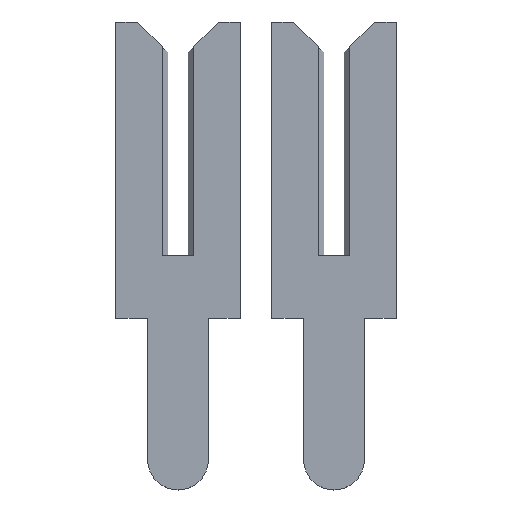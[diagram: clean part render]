
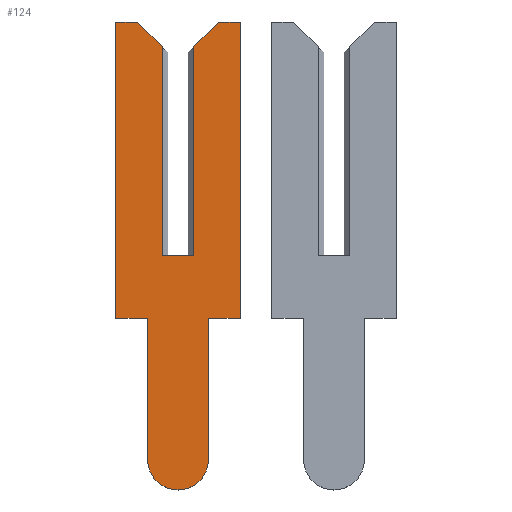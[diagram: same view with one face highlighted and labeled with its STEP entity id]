
A CAD part, top view. The second image highlights one B-rep face of the part: STEP entity #124.
In plain terms, the highlighted face is planar.
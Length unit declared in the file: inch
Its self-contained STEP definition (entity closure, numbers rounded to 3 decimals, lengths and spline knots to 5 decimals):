
#14 = ORIENTED_EDGE ( 'NONE', *, *, #624, .F. ) ;
#21 = VERTEX_POINT ( 'NONE', #596 ) ;
#33 = DIRECTION ( 'NONE',  ( 0., -0.707, 0.707 ) ) ;
#43 = EDGE_CURVE ( 'NONE', #848, #431, #293, .T. ) ;
#51 = VECTOR ( 'NONE', #459, 39.37008 ) ;
#69 = ORIENTED_EDGE ( 'NONE', *, *, #157, .F. ) ;
#72 = VERTEX_POINT ( 'NONE', #143 ) ;
#75 = VECTOR ( 'NONE', #466, 39.37008 ) ;
#78 = DIRECTION ( 'NONE',  ( 0., -1., 0. ) ) ;
#87 = VERTEX_POINT ( 'NONE', #483 ) ;
#93 = VERTEX_POINT ( 'NONE', #812 ) ;
#108 = CARTESIAN_POINT ( 'NONE',  ( -0.01, 0., 0.01 ) ) ;
#117 = ORIENTED_EDGE ( 'NONE', *, *, #424, .F. ) ;
#119 = VECTOR ( 'NONE', #715, 39.37008 ) ;
#124 = ADVANCED_FACE ( 'NONE', ( #819 ), #273, .F. ) ;
#130 = AXIS2_PLACEMENT_3D ( 'NONE', #264, #809, #267 ) ;
#131 = CARTESIAN_POINT ( 'NONE',  ( -0.01, 0., 0.0065 ) ) ;
#134 = CARTESIAN_POINT ( 'NONE',  ( -0.01, -0.04, 0.04 ) ) ;
#137 = EDGE_CURVE ( 'NONE', #21, #760, #778, .T. ) ;
#143 = CARTESIAN_POINT ( 'NONE',  ( -0.01, -0.1305, -0.0195 ) ) ;
#151 = VECTOR ( 'NONE', #699, 39.37008 ) ;
#154 = ORIENTED_EDGE ( 'NONE', *, *, #754, .F. ) ;
#157 = EDGE_CURVE ( 'NONE', #214, #307, #317, .T. ) ;
#164 = ORIENTED_EDGE ( 'NONE', *, *, #43, .T. ) ;
#190 = LINE ( 'NONE', #434, #850 ) ;
#195 = CARTESIAN_POINT ( 'NONE',  ( -0.01, -0.04, 0.0195 ) ) ;
#204 = CARTESIAN_POINT ( 'NONE',  ( -0.01, 0.134, -0.01 ) ) ;
#213 = CARTESIAN_POINT ( 'NONE',  ( -0.01, 0.15, -0.04 ) ) ;
#214 = VERTEX_POINT ( 'NONE', #550 ) ;
#228 = VECTOR ( 'NONE', #33, 39.37008 ) ;
#243 = DIRECTION ( 'NONE',  ( 0., 0., 1. ) ) ;
#245 = ORIENTED_EDGE ( 'NONE', *, *, #669, .F. ) ;
#247 = EDGE_CURVE ( 'NONE', #848, #87, #341, .T. ) ;
#249 = VECTOR ( 'NONE', #499, 39.37008 ) ;
#256 = EDGE_CURVE ( 'NONE', #72, #265, #190, .T. ) ;
#261 = ORIENTED_EDGE ( 'NONE', *, *, #315, .F. ) ;
#262 = CARTESIAN_POINT ( 'NONE',  ( -0.01, -0.04, -0.04 ) ) ;
#264 = CARTESIAN_POINT ( 'NONE',  ( -0.01, -0.1305, 0. ) ) ;
#265 = VERTEX_POINT ( 'NONE', #546 ) ;
#267 = DIRECTION ( 'NONE',  ( 0., 0., -1. ) ) ;
#272 = LINE ( 'NONE', #131, #601 ) ;
#273 = PLANE ( 'NONE',  #782 ) ;
#283 = VECTOR ( 'NONE', #592, 39.37008 ) ;
#288 = CARTESIAN_POINT ( 'NONE',  ( -0.01, 0.1305, 0.0065 ) ) ;
#293 = LINE ( 'NONE', #815, #657 ) ;
#307 = VERTEX_POINT ( 'NONE', #636 ) ;
#308 = CARTESIAN_POINT ( 'NONE',  ( -0.01, -0.04, 0.0195 ) ) ;
#315 = EDGE_CURVE ( 'NONE', #491, #589, #570, .T. ) ;
#317 = LINE ( 'NONE', #768, #249 ) ;
#326 = CARTESIAN_POINT ( 'NONE',  ( -0.01, 0.15, 0.026 ) ) ;
#330 = LINE ( 'NONE', #134, #283 ) ;
#337 = ORIENTED_EDGE ( 'NONE', *, *, #718, .F. ) ;
#338 = DIRECTION ( 'NONE',  ( 0., 0., 1. ) ) ;
#341 = LINE ( 'NONE', #288, #151 ) ;
#344 = DIRECTION ( 'NONE',  ( 0., 1., 0. ) ) ;
#360 = CARTESIAN_POINT ( 'NONE',  ( -0.01, 0.1305, -0.0065 ) ) ;
#393 = VECTOR ( 'NONE', #344, 39.37008 ) ;
#414 = DIRECTION ( 'NONE',  ( 1., 0., 0. ) ) ;
#417 = ORIENTED_EDGE ( 'NONE', *, *, #137, .F. ) ;
#424 = EDGE_CURVE ( 'NONE', #721, #21, #678, .T. ) ;
#431 = VERTEX_POINT ( 'NONE', #108 ) ;
#434 = CARTESIAN_POINT ( 'NONE',  ( -0.01, -0.04, -0.0195 ) ) ;
#443 = VECTOR ( 'NONE', #471, 39.37008 ) ;
#459 = DIRECTION ( 'NONE',  ( 0., 0., 1. ) ) ;
#466 = DIRECTION ( 'NONE',  ( 0., -1., 0. ) ) ;
#471 = DIRECTION ( 'NONE',  ( 0., 0., -1. ) ) ;
#480 = CIRCLE ( 'NONE', #130, 0.0195 ) ;
#481 = EDGE_CURVE ( 'NONE', #87, #214, #727, .T. ) ;
#483 = CARTESIAN_POINT ( 'NONE',  ( -0.01, 0.15, 0.026 ) ) ;
#491 = VERTEX_POINT ( 'NONE', #195 ) ;
#499 = DIRECTION ( 'NONE',  ( 0., -1., 0. ) ) ;
#527 = CARTESIAN_POINT ( 'NONE',  ( -0.01, -0.1305, -0.01 ) ) ;
#546 = CARTESIAN_POINT ( 'NONE',  ( -0.01, -0.04, -0.0195 ) ) ;
#550 = CARTESIAN_POINT ( 'NONE',  ( -0.01, 0.15, 0.04 ) ) ;
#556 = DIRECTION ( 'NONE',  ( 0., 1., 0. ) ) ;
#570 = LINE ( 'NONE', #308, #119 ) ;
#589 = VERTEX_POINT ( 'NONE', #853 ) ;
#592 = DIRECTION ( 'NONE',  ( 0., 0., -1. ) ) ;
#596 = CARTESIAN_POINT ( 'NONE',  ( -0.01, 0.15, -0.026 ) ) ;
#601 = VECTOR ( 'NONE', #338, 39.37008 ) ;
#606 = DIRECTION ( 'NONE',  ( 0., 0., -1. ) ) ;
#615 = CARTESIAN_POINT ( 'NONE',  ( -0.01, 0.134, 0.01 ) ) ;
#617 = EDGE_CURVE ( 'NONE', #786, #431, #272, .T. ) ;
#623 = ORIENTED_EDGE ( 'NONE', *, *, #247, .F. ) ;
#624 = EDGE_CURVE ( 'NONE', #93, #721, #839, .T. ) ;
#632 = CARTESIAN_POINT ( 'NONE',  ( -0.01, 0.15, -0.026 ) ) ;
#636 = CARTESIAN_POINT ( 'NONE',  ( -0.01, -0.04, 0.04 ) ) ;
#638 = LINE ( 'NONE', #262, #443 ) ;
#639 = ORIENTED_EDGE ( 'NONE', *, *, #481, .F. ) ;
#642 = ORIENTED_EDGE ( 'NONE', *, *, #617, .F. ) ;
#655 = ORIENTED_EDGE ( 'NONE', *, *, #256, .F. ) ;
#657 = VECTOR ( 'NONE', #78, 39.37008 ) ;
#664 = CARTESIAN_POINT ( 'NONE',  ( -0.01, 0.15, -0.04 ) ) ;
#666 = ORIENTED_EDGE ( 'NONE', *, *, #764, .F. ) ;
#669 = EDGE_CURVE ( 'NONE', #589, #72, #480, .T. ) ;
#676 = LINE ( 'NONE', #527, #75 ) ;
#678 = LINE ( 'NONE', #632, #769 ) ;
#699 = DIRECTION ( 'NONE',  ( 0., 0.707, 0.707 ) ) ;
#715 = DIRECTION ( 'NONE',  ( 0., -1., 0. ) ) ;
#718 = EDGE_CURVE ( 'NONE', #760, #786, #676, .T. ) ;
#721 = VERTEX_POINT ( 'NONE', #213 ) ;
#727 = LINE ( 'NONE', #326, #51 ) ;
#733 = CARTESIAN_POINT ( 'NONE',  ( -0.01, 0., -0.01 ) ) ;
#740 = CARTESIAN_POINT ( 'NONE',  ( -0.01, -0.1305, 0. ) ) ;
#754 = EDGE_CURVE ( 'NONE', #307, #491, #330, .T. ) ;
#760 = VERTEX_POINT ( 'NONE', #204 ) ;
#764 = EDGE_CURVE ( 'NONE', #265, #93, #638, .T. ) ;
#768 = CARTESIAN_POINT ( 'NONE',  ( -0.01, 0.15, 0.04 ) ) ;
#769 = VECTOR ( 'NONE', #243, 39.37008 ) ;
#778 = LINE ( 'NONE', #360, #228 ) ;
#779 = EDGE_LOOP ( 'NONE', ( #164, #642, #337, #417, #117, #14, #666, #655, #245, #261, #154, #69, #639, #623 ) ) ;
#782 = AXIS2_PLACEMENT_3D ( 'NONE', #740, #414, #606 ) ;
#786 = VERTEX_POINT ( 'NONE', #733 ) ;
#809 = DIRECTION ( 'NONE',  ( 1., 0., 0. ) ) ;
#812 = CARTESIAN_POINT ( 'NONE',  ( -0.01, -0.04, -0.04 ) ) ;
#815 = CARTESIAN_POINT ( 'NONE',  ( -0.01, 0.15, 0.01 ) ) ;
#819 = FACE_OUTER_BOUND ( 'NONE', #779, .T. ) ;
#839 = LINE ( 'NONE', #664, #393 ) ;
#848 = VERTEX_POINT ( 'NONE', #615 ) ;
#850 = VECTOR ( 'NONE', #556, 39.37008 ) ;
#853 = CARTESIAN_POINT ( 'NONE',  ( -0.01, -0.1305, 0.0195 ) ) ;
